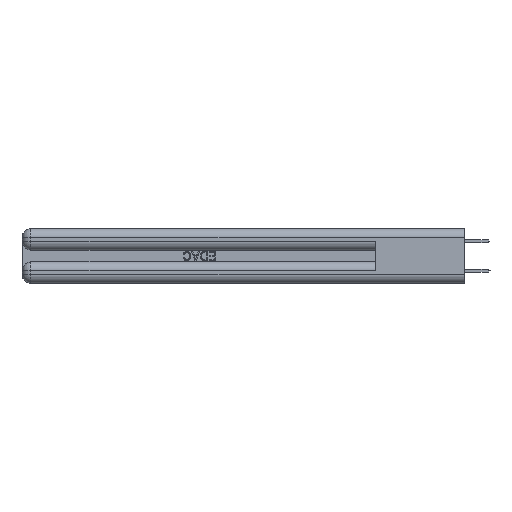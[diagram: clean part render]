
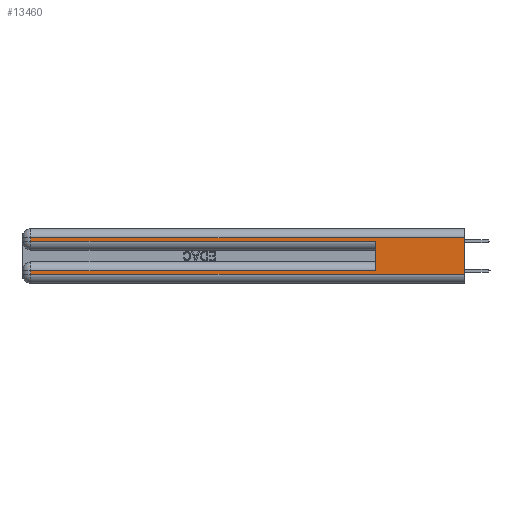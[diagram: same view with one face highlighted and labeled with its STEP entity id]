
A CAD part, left-side view. The second image highlights one B-rep face of the part: STEP entity #13460.
In plain terms, the highlighted planar face has unit normal (-1, 0, 0).
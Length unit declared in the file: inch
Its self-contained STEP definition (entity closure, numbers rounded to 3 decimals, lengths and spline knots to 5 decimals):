
#260 = VERTEX_POINT ( 'NONE', #19825 ) ;
#2161 = VECTOR ( 'NONE', #27564, 39.37008 ) ;
#2949 = VECTOR ( 'NONE', #33652, 39.37008 ) ;
#4454 = DIRECTION ( 'NONE',  ( 0., 0., 1. ) ) ;
#4707 = LINE ( 'NONE', #31424, #39380 ) ;
#5384 = VERTEX_POINT ( 'NONE', #24301 ) ;
#6791 = ORIENTED_EDGE ( 'NONE', *, *, #41558, .T. ) ;
#8009 = EDGE_CURVE ( 'NONE', #42009, #37188, #35030, .T. ) ;
#8256 = CARTESIAN_POINT ( 'NONE',  ( 0., 0.6, 0.285 ) ) ;
#8359 = VECTOR ( 'NONE', #16312, 39.37008 ) ;
#8650 = CARTESIAN_POINT ( 'NONE',  ( 0., 2.94, 0.085 ) ) ;
#9509 = CARTESIAN_POINT ( 'NONE',  ( 0., 0., 0.31 ) ) ;
#9944 = DIRECTION ( 'NONE',  ( 0., 0., -1. ) ) ;
#10969 = LINE ( 'NONE', #19961, #8359 ) ;
#11551 = CARTESIAN_POINT ( 'NONE',  ( 0., 2.94, 0.285 ) ) ;
#12089 = EDGE_CURVE ( 'NONE', #37188, #260, #25868, .T. ) ;
#12844 = CARTESIAN_POINT ( 'NONE',  ( 0., 0., 0.37 ) ) ;
#13460 = ADVANCED_FACE ( 'NONE', ( #35167 ), #18078, .F. ) ;
#14454 = DIRECTION ( 'NONE',  ( 1., 0., 0. ) ) ;
#16048 = LINE ( 'NONE', #30164, #25535 ) ;
#16312 = DIRECTION ( 'NONE',  ( 0., 0., -1. ) ) ;
#18078 = PLANE ( 'NONE',  #19729 ) ;
#18206 = ORIENTED_EDGE ( 'NONE', *, *, #32532, .F. ) ;
#19715 = ORIENTED_EDGE ( 'NONE', *, *, #36070, .T. ) ;
#19729 = AXIS2_PLACEMENT_3D ( 'NONE', #31650, #14454, #38033 ) ;
#19825 = CARTESIAN_POINT ( 'NONE',  ( 0., 2.94, 0.06 ) ) ;
#19830 = DIRECTION ( 'NONE',  ( 0., 1., 0. ) ) ;
#19961 = CARTESIAN_POINT ( 'NONE',  ( 0., 2.94, 0.37 ) ) ;
#20141 = CARTESIAN_POINT ( 'NONE',  ( 0., 0., 0.06 ) ) ;
#21773 = VERTEX_POINT ( 'NONE', #8256 ) ;
#24301 = CARTESIAN_POINT ( 'NONE',  ( 0., 2.94, 0.31 ) ) ;
#24832 = CARTESIAN_POINT ( 'NONE',  ( 0., 0., 0.285 ) ) ;
#25535 = VECTOR ( 'NONE', #19830, 39.37008 ) ;
#25557 = EDGE_CURVE ( 'NONE', #260, #43008, #4707, .T. ) ;
#25868 = LINE ( 'NONE', #26733, #2161 ) ;
#26733 = CARTESIAN_POINT ( 'NONE',  ( 0., 2.94, 0.37 ) ) ;
#26761 = ORIENTED_EDGE ( 'NONE', *, *, #25557, .T. ) ;
#27271 = VERTEX_POINT ( 'NONE', #11551 ) ;
#27522 = EDGE_CURVE ( 'NONE', #42009, #21773, #32575, .T. ) ;
#27564 = DIRECTION ( 'NONE',  ( 0., 0., -1. ) ) ;
#27966 = ORIENTED_EDGE ( 'NONE', *, *, #12089, .T. ) ;
#29908 = EDGE_LOOP ( 'NONE', ( #18206, #33313, #6791, #19715, #32850, #34857, #27966, #26761 ) ) ;
#30164 = CARTESIAN_POINT ( 'NONE',  ( 0., 0., 0.31 ) ) ;
#30976 = VECTOR ( 'NONE', #4454, 39.37008 ) ;
#31175 = EDGE_CURVE ( 'NONE', #37896, #5384, #16048, .T. ) ;
#31412 = DIRECTION ( 'NONE',  ( 0., -1., 0. ) ) ;
#31424 = CARTESIAN_POINT ( 'NONE',  ( 0., 0., 0.06 ) ) ;
#31650 = CARTESIAN_POINT ( 'NONE',  ( 0., 0., 0.37 ) ) ;
#32532 = EDGE_CURVE ( 'NONE', #37896, #43008, #35382, .T. ) ;
#32575 = LINE ( 'NONE', #41412, #30976 ) ;
#32850 = ORIENTED_EDGE ( 'NONE', *, *, #27522, .F. ) ;
#33313 = ORIENTED_EDGE ( 'NONE', *, *, #31175, .T. ) ;
#33652 = DIRECTION ( 'NONE',  ( 0., 1., 0. ) ) ;
#34857 = ORIENTED_EDGE ( 'NONE', *, *, #8009, .T. ) ;
#35030 = LINE ( 'NONE', #39949, #2949 ) ;
#35167 = FACE_OUTER_BOUND ( 'NONE', #29908, .T. ) ;
#35382 = LINE ( 'NONE', #12844, #42694 ) ;
#36070 = EDGE_CURVE ( 'NONE', #27271, #21773, #40753, .T. ) ;
#37125 = VECTOR ( 'NONE', #31412, 39.37008 ) ;
#37188 = VERTEX_POINT ( 'NONE', #8650 ) ;
#37896 = VERTEX_POINT ( 'NONE', #9509 ) ;
#38033 = DIRECTION ( 'NONE',  ( 0., 0., -1. ) ) ;
#38689 = CARTESIAN_POINT ( 'NONE',  ( 0., 0.6, 0.085 ) ) ;
#39380 = VECTOR ( 'NONE', #41348, 39.37008 ) ;
#39949 = CARTESIAN_POINT ( 'NONE',  ( 0., 0., 0.085 ) ) ;
#40753 = LINE ( 'NONE', #24832, #37125 ) ;
#41348 = DIRECTION ( 'NONE',  ( 0., -1., 0. ) ) ;
#41412 = CARTESIAN_POINT ( 'NONE',  ( 0., 0.6, 0.145 ) ) ;
#41558 = EDGE_CURVE ( 'NONE', #5384, #27271, #10969, .T. ) ;
#42009 = VERTEX_POINT ( 'NONE', #38689 ) ;
#42694 = VECTOR ( 'NONE', #9944, 39.37008 ) ;
#43008 = VERTEX_POINT ( 'NONE', #20141 ) ;
